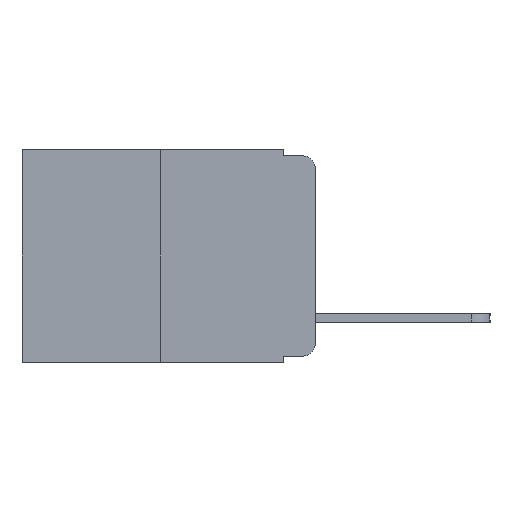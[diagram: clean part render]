
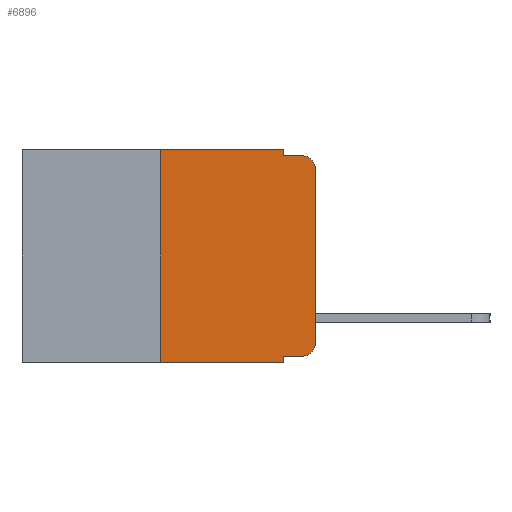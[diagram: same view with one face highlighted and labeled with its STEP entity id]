
A CAD part, left-side view. The second image highlights one B-rep face of the part: STEP entity #6896.
In plain terms, the highlighted planar face has unit normal (-1, 0, 0).
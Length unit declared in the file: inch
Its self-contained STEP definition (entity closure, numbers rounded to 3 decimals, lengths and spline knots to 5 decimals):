
#79 = ORIENTED_EDGE ( 'NONE', *, *, #4926, .F. ) ;
#189 = VERTEX_POINT ( 'NONE', #6932 ) ;
#207 = VECTOR ( 'NONE', #979, 39.37008 ) ;
#376 = CARTESIAN_POINT ( 'NONE',  ( 0., 0.051, -0.333 ) ) ;
#406 = ORIENTED_EDGE ( 'NONE', *, *, #759, .F. ) ;
#415 = ORIENTED_EDGE ( 'NONE', *, *, #12306, .F. ) ;
#524 = VECTOR ( 'NONE', #6054, 39.37008 ) ;
#594 = CIRCLE ( 'NONE', #3325, 0.02 ) ;
#759 = EDGE_CURVE ( 'NONE', #4601, #2994, #3320, .T. ) ;
#876 = LINE ( 'NONE', #10785, #524 ) ;
#958 = DIRECTION ( 'NONE',  ( 0., -1., 0. ) ) ;
#979 = DIRECTION ( 'NONE',  ( 0., 0., -1. ) ) ;
#991 = FACE_OUTER_BOUND ( 'NONE', #1638, .T. ) ;
#997 = CARTESIAN_POINT ( 'NONE',  ( 0., 0.051, 0. ) ) ;
#1080 = CARTESIAN_POINT ( 'NONE',  ( 0., 0.02, -0.313 ) ) ;
#1448 = VERTEX_POINT ( 'NONE', #8575 ) ;
#1449 = CARTESIAN_POINT ( 'NONE',  ( 0., 0.02, -0.333 ) ) ;
#1520 = EDGE_CURVE ( 'NONE', #2994, #2647, #3820, .T. ) ;
#1638 = EDGE_LOOP ( 'NONE', ( #7623, #2305, #7112, #406, #79, #415, #4981, #7906, #7639, #9055 ) ) ;
#1967 = DIRECTION ( 'NONE',  ( 0., 0., 1. ) ) ;
#2077 = DIRECTION ( 'NONE',  ( 0., 0., -1. ) ) ;
#2110 = EDGE_CURVE ( 'NONE', #5066, #2647, #4813, .T. ) ;
#2305 = ORIENTED_EDGE ( 'NONE', *, *, #2110, .T. ) ;
#2314 = CARTESIAN_POINT ( 'NONE',  ( 0., 0.051, -0.01 ) ) ;
#2388 = CARTESIAN_POINT ( 'NONE',  ( 0., 0.02, -0.01 ) ) ;
#2503 = DIRECTION ( 'NONE',  ( 0., 0., 1. ) ) ;
#2647 = VERTEX_POINT ( 'NONE', #2388 ) ;
#2653 = CARTESIAN_POINT ( 'NONE',  ( 0., 0.473, 0. ) ) ;
#2765 = EDGE_CURVE ( 'NONE', #189, #5066, #5822, .T. ) ;
#2928 = LINE ( 'NONE', #10469, #207 ) ;
#2938 = VECTOR ( 'NONE', #12303, 39.37008 ) ;
#2994 = VERTEX_POINT ( 'NONE', #12122 ) ;
#3050 = CARTESIAN_POINT ( 'NONE',  ( 0., 0.051, -0.343 ) ) ;
#3198 = VECTOR ( 'NONE', #958, 39.37008 ) ;
#3320 = LINE ( 'NONE', #6290, #12297 ) ;
#3325 = AXIS2_PLACEMENT_3D ( 'NONE', #1080, #7775, #2077 ) ;
#3331 = VECTOR ( 'NONE', #2503, 39.37008 ) ;
#3388 = CARTESIAN_POINT ( 'NONE',  ( 0., 0.25, 0. ) ) ;
#3604 = DIRECTION ( 'NONE',  ( 0., 0., -1. ) ) ;
#3820 = LINE ( 'NONE', #2314, #3198 ) ;
#3998 = CARTESIAN_POINT ( 'NONE',  ( 0., 0.473, -0.343 ) ) ;
#4222 = VECTOR ( 'NONE', #4296, 39.37008 ) ;
#4296 = DIRECTION ( 'NONE',  ( 0., -1., 0. ) ) ;
#4516 = CARTESIAN_POINT ( 'NONE',  ( 0., 0.02, -0.03 ) ) ;
#4601 = VERTEX_POINT ( 'NONE', #997 ) ;
#4813 = CIRCLE ( 'NONE', #6100, 0.02 ) ;
#4926 = EDGE_CURVE ( 'NONE', #6528, #4601, #876, .T. ) ;
#4981 = ORIENTED_EDGE ( 'NONE', *, *, #9994, .T. ) ;
#5066 = VERTEX_POINT ( 'NONE', #8215 ) ;
#5448 = LINE ( 'NONE', #3998, #2938 ) ;
#5822 = LINE ( 'NONE', #8894, #3331 ) ;
#6054 = DIRECTION ( 'NONE',  ( 0., -1., 0. ) ) ;
#6100 = AXIS2_PLACEMENT_3D ( 'NONE', #4516, #9551, #7477 ) ;
#6290 = CARTESIAN_POINT ( 'NONE',  ( 0., 0.051, 0. ) ) ;
#6528 = VERTEX_POINT ( 'NONE', #3388 ) ;
#6665 = VERTEX_POINT ( 'NONE', #6687 ) ;
#6687 = CARTESIAN_POINT ( 'NONE',  ( 0., 0.051, -0.333 ) ) ;
#6896 = ADVANCED_FACE ( 'NONE', ( #991 ), #8324, .F. ) ;
#6932 = CARTESIAN_POINT ( 'NONE',  ( 0., 0., -0.313 ) ) ;
#7112 = ORIENTED_EDGE ( 'NONE', *, *, #1520, .F. ) ;
#7477 = DIRECTION ( 'NONE',  ( 0., 0., -1. ) ) ;
#7623 = ORIENTED_EDGE ( 'NONE', *, *, #2765, .T. ) ;
#7639 = ORIENTED_EDGE ( 'NONE', *, *, #11725, .T. ) ;
#7775 = DIRECTION ( 'NONE',  ( -1., 0., 0. ) ) ;
#7906 = ORIENTED_EDGE ( 'NONE', *, *, #10583, .F. ) ;
#8215 = CARTESIAN_POINT ( 'NONE',  ( 0., 0., -0.03 ) ) ;
#8292 = DIRECTION ( 'NONE',  ( 1., 0., 0. ) ) ;
#8324 = PLANE ( 'NONE',  #11225 ) ;
#8482 = VERTEX_POINT ( 'NONE', #3050 ) ;
#8575 = CARTESIAN_POINT ( 'NONE',  ( 0., 0.25, -0.343 ) ) ;
#8894 = CARTESIAN_POINT ( 'NONE',  ( 0., 0., 0. ) ) ;
#9055 = ORIENTED_EDGE ( 'NONE', *, *, #9951, .T. ) ;
#9285 = LINE ( 'NONE', #12178, #11365 ) ;
#9297 = LINE ( 'NONE', #376, #4222 ) ;
#9551 = DIRECTION ( 'NONE',  ( -1., 0., 0. ) ) ;
#9951 = EDGE_CURVE ( 'NONE', #10933, #189, #594, .T. ) ;
#9994 = EDGE_CURVE ( 'NONE', #1448, #8482, #5448, .T. ) ;
#10236 = DIRECTION ( 'NONE',  ( 0., 0., -1. ) ) ;
#10469 = CARTESIAN_POINT ( 'NONE',  ( 0., 0.051, 0. ) ) ;
#10583 = EDGE_CURVE ( 'NONE', #6665, #8482, #2928, .T. ) ;
#10785 = CARTESIAN_POINT ( 'NONE',  ( 0., 0.473, 0. ) ) ;
#10933 = VERTEX_POINT ( 'NONE', #1449 ) ;
#11225 = AXIS2_PLACEMENT_3D ( 'NONE', #2653, #8292, #3604 ) ;
#11365 = VECTOR ( 'NONE', #1967, 39.37008 ) ;
#11725 = EDGE_CURVE ( 'NONE', #6665, #10933, #9297, .T. ) ;
#12122 = CARTESIAN_POINT ( 'NONE',  ( 0., 0.051, -0.01 ) ) ;
#12178 = CARTESIAN_POINT ( 'NONE',  ( 0., 0.25, 0. ) ) ;
#12297 = VECTOR ( 'NONE', #10236, 39.37008 ) ;
#12303 = DIRECTION ( 'NONE',  ( 0., -1., 0. ) ) ;
#12306 = EDGE_CURVE ( 'NONE', #1448, #6528, #9285, .T. ) ;
